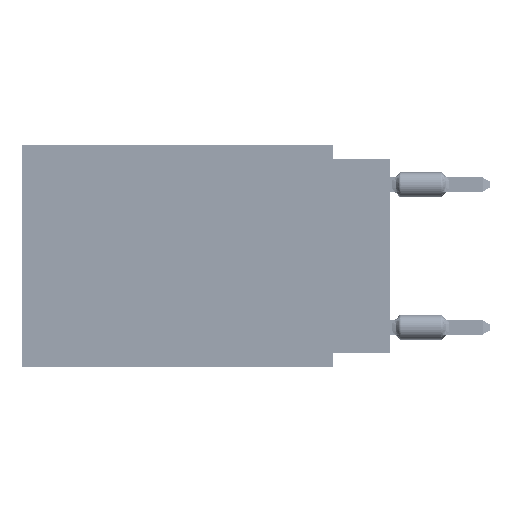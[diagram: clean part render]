
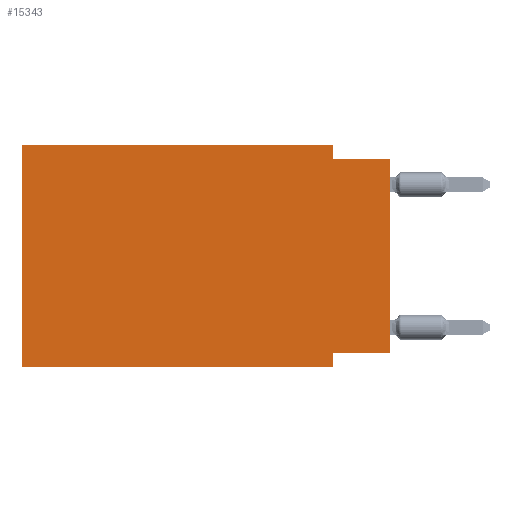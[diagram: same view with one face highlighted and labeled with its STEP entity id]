
A CAD part, left-side view. The second image highlights one B-rep face of the part: STEP entity #15343.
In plain terms, the highlighted planar face has unit normal (-1, 0, 0).
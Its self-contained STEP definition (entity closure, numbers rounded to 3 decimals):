
#555 = CARTESIAN_POINT ( 'NONE',  ( 0., 0., -9.271 ) ) ;
#4393 = VECTOR ( 'NONE', #62141, 1000. ) ;
#4605 = CARTESIAN_POINT ( 'NONE',  ( 0., 16.383, -9.906 ) ) ;
#4729 = CARTESIAN_POINT ( 'NONE',  ( 0., 16.383, 0. ) ) ;
#5227 = VERTEX_POINT ( 'NONE', #17102 ) ;
#5636 = PLANE ( 'NONE',  #11760 ) ;
#6223 = VERTEX_POINT ( 'NONE', #60486 ) ;
#7231 = CARTESIAN_POINT ( 'NONE',  ( 0., 2.54, 0. ) ) ;
#7264 = VECTOR ( 'NONE', #33959, 1000. ) ;
#7283 = CARTESIAN_POINT ( 'NONE',  ( 0., 2.54, 0. ) ) ;
#7551 = CARTESIAN_POINT ( 'NONE',  ( 0., 0., -9.271 ) ) ;
#8991 = DIRECTION ( 'NONE',  ( 0., 0., -1. ) ) ;
#9038 = EDGE_CURVE ( 'NONE', #6223, #22835, #25174, .T. ) ;
#9496 = VERTEX_POINT ( 'NONE', #55295 ) ;
#10203 = CARTESIAN_POINT ( 'NONE',  ( 0., 16.383, 0. ) ) ;
#11028 = DIRECTION ( 'NONE',  ( 0., -1., 0. ) ) ;
#11226 = CARTESIAN_POINT ( 'NONE',  ( 0., 0., -0.635 ) ) ;
#11760 = AXIS2_PLACEMENT_3D ( 'NONE', #57415, #52273, #26201 ) ;
#13672 = CARTESIAN_POINT ( 'NONE',  ( 0., 0., 0. ) ) ;
#14135 = CARTESIAN_POINT ( 'NONE',  ( 0., 2.54, -9.906 ) ) ;
#15343 = ADVANCED_FACE ( 'NONE', ( #21391 ), #5636, .F. ) ;
#15655 = EDGE_CURVE ( 'NONE', #5227, #22835, #18944, .T. ) ;
#15946 = EDGE_CURVE ( 'NONE', #55481, #9496, #54229, .T. ) ;
#16173 = LINE ( 'NONE', #30935, #58440 ) ;
#16368 = ORIENTED_EDGE ( 'NONE', *, *, #15946, .F. ) ;
#17102 = CARTESIAN_POINT ( 'NONE',  ( 0., 2.54, -9.271 ) ) ;
#17181 = DIRECTION ( 'NONE',  ( 0., 0., -1. ) ) ;
#18944 = LINE ( 'NONE', #14135, #36380 ) ;
#20275 = CARTESIAN_POINT ( 'NONE',  ( 0., 16.383, 0. ) ) ;
#20825 = ORIENTED_EDGE ( 'NONE', *, *, #49030, .F. ) ;
#21391 = FACE_OUTER_BOUND ( 'NONE', #42606, .T. ) ;
#22835 = VERTEX_POINT ( 'NONE', #28621 ) ;
#24417 = LINE ( 'NONE', #20275, #4393 ) ;
#25174 = LINE ( 'NONE', #4605, #64922 ) ;
#26201 = DIRECTION ( 'NONE',  ( 0., 0., -1. ) ) ;
#26982 = VERTEX_POINT ( 'NONE', #555 ) ;
#28621 = CARTESIAN_POINT ( 'NONE',  ( 0., 2.54, -9.906 ) ) ;
#29137 = LINE ( 'NONE', #7551, #7264 ) ;
#30896 = VECTOR ( 'NONE', #17181, 1000. ) ;
#30935 = CARTESIAN_POINT ( 'NONE',  ( 0., 0., -0.635 ) ) ;
#33959 = DIRECTION ( 'NONE',  ( 0., 1., 0. ) ) ;
#34623 = DIRECTION ( 'NONE',  ( 0., 0., 1. ) ) ;
#34749 = VERTEX_POINT ( 'NONE', #11226 ) ;
#36380 = VECTOR ( 'NONE', #8991, 1000. ) ;
#40232 = ORIENTED_EDGE ( 'NONE', *, *, #42290, .F. ) ;
#40610 = DIRECTION ( 'NONE',  ( 0., -1., 0. ) ) ;
#41728 = ORIENTED_EDGE ( 'NONE', *, *, #51557, .F. ) ;
#42290 = EDGE_CURVE ( 'NONE', #6223, #47756, #24417, .T. ) ;
#42606 = EDGE_LOOP ( 'NONE', ( #62509, #41728, #16368, #20825, #40232, #60878, #64768, #56446 ) ) ;
#47756 = VERTEX_POINT ( 'NONE', #4729 ) ;
#49030 = EDGE_CURVE ( 'NONE', #47756, #55481, #52407, .T. ) ;
#51557 = EDGE_CURVE ( 'NONE', #9496, #34749, #16173, .T. ) ;
#52068 = DIRECTION ( 'NONE',  ( 0., -1., 0. ) ) ;
#52273 = DIRECTION ( 'NONE',  ( 1., 0., 0. ) ) ;
#52407 = LINE ( 'NONE', #10203, #52773 ) ;
#52773 = VECTOR ( 'NONE', #52068, 1000. ) ;
#53725 = VECTOR ( 'NONE', #34623, 1000. ) ;
#54229 = LINE ( 'NONE', #7231, #30896 ) ;
#55295 = CARTESIAN_POINT ( 'NONE',  ( 0., 2.54, -0.635 ) ) ;
#55481 = VERTEX_POINT ( 'NONE', #7283 ) ;
#56446 = ORIENTED_EDGE ( 'NONE', *, *, #57161, .F. ) ;
#57161 = EDGE_CURVE ( 'NONE', #26982, #5227, #29137, .T. ) ;
#57415 = CARTESIAN_POINT ( 'NONE',  ( 0., 16.383, 0. ) ) ;
#58440 = VECTOR ( 'NONE', #11028, 1000. ) ;
#60486 = CARTESIAN_POINT ( 'NONE',  ( 0., 16.383, -9.906 ) ) ;
#60878 = ORIENTED_EDGE ( 'NONE', *, *, #9038, .T. ) ;
#62141 = DIRECTION ( 'NONE',  ( 0., 0., 1. ) ) ;
#62509 = ORIENTED_EDGE ( 'NONE', *, *, #63540, .T. ) ;
#63540 = EDGE_CURVE ( 'NONE', #26982, #34749, #66169, .T. ) ;
#64768 = ORIENTED_EDGE ( 'NONE', *, *, #15655, .F. ) ;
#64922 = VECTOR ( 'NONE', #40610, 1000. ) ;
#66169 = LINE ( 'NONE', #13672, #53725 ) ;
